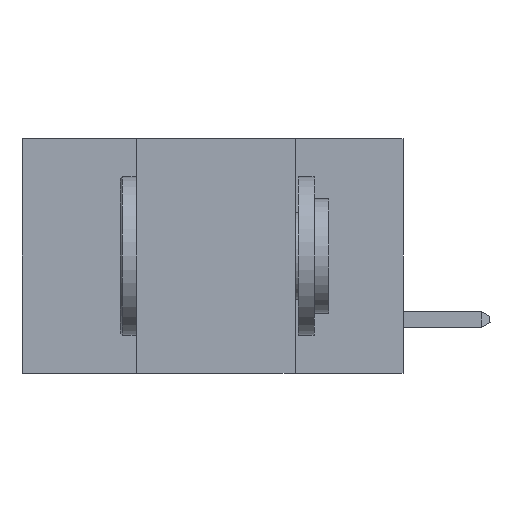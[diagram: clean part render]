
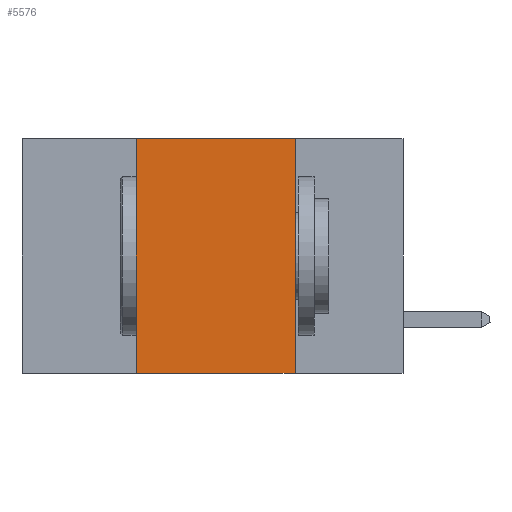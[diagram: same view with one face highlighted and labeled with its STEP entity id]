
A CAD part, left-side view. The second image highlights one B-rep face of the part: STEP entity #5576.
In plain terms, the highlighted planar face has unit normal (-1, 0, 0).
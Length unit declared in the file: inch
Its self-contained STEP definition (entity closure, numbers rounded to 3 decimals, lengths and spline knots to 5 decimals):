
#89 = VERTEX_POINT ( 'NONE', #5878 ) ;
#195 = CARTESIAN_POINT ( 'NONE',  ( 0., 0.6, -0.37 ) ) ;
#388 = VECTOR ( 'NONE', #3309, 39.37008 ) ;
#470 = PLANE ( 'NONE',  #1290 ) ;
#538 = VECTOR ( 'NONE', #8555, 39.37008 ) ;
#962 = LINE ( 'NONE', #195, #388 ) ;
#1290 = AXIS2_PLACEMENT_3D ( 'NONE', #4885, #7760, #3358 ) ;
#1533 = ORIENTED_EDGE ( 'NONE', *, *, #8384, .T. ) ;
#1675 = DIRECTION ( 'NONE',  ( 0., 0., -1. ) ) ;
#1968 = VECTOR ( 'NONE', #2813, 39.37008 ) ;
#2813 = DIRECTION ( 'NONE',  ( 0., -1., 0. ) ) ;
#2861 = VERTEX_POINT ( 'NONE', #6689 ) ;
#2905 = ORIENTED_EDGE ( 'NONE', *, *, #6651, .F. ) ;
#3309 = DIRECTION ( 'NONE',  ( 0., -1., 0. ) ) ;
#3358 = DIRECTION ( 'NONE',  ( 0., 0., -1. ) ) ;
#4235 = EDGE_LOOP ( 'NONE', ( #5993, #7363, #2905, #1533 ) ) ;
#4421 = LINE ( 'NONE', #8132, #1968 ) ;
#4524 = CARTESIAN_POINT ( 'NONE',  ( 0., 0.42, -0.37 ) ) ;
#4829 = CARTESIAN_POINT ( 'NONE',  ( 0., 0.42, 0. ) ) ;
#4885 = CARTESIAN_POINT ( 'NONE',  ( 0., 0.6, 0. ) ) ;
#5033 = VERTEX_POINT ( 'NONE', #4524 ) ;
#5075 = VERTEX_POINT ( 'NONE', #9316 ) ;
#5366 = EDGE_CURVE ( 'NONE', #2861, #89, #7526, .T. ) ;
#5576 = ADVANCED_FACE ( 'NONE', ( #6583 ), #470, .F. ) ;
#5878 = CARTESIAN_POINT ( 'NONE',  ( 0., 0.17, -0.37 ) ) ;
#5993 = ORIENTED_EDGE ( 'NONE', *, *, #5366, .F. ) ;
#6510 = LINE ( 'NONE', #4829, #538 ) ;
#6583 = FACE_OUTER_BOUND ( 'NONE', #4235, .T. ) ;
#6651 = EDGE_CURVE ( 'NONE', #5033, #5075, #6510, .T. ) ;
#6689 = CARTESIAN_POINT ( 'NONE',  ( 0., 0.17, 0. ) ) ;
#7363 = ORIENTED_EDGE ( 'NONE', *, *, #8908, .F. ) ;
#7526 = LINE ( 'NONE', #8982, #9149 ) ;
#7760 = DIRECTION ( 'NONE',  ( 1., 0., 0. ) ) ;
#8132 = CARTESIAN_POINT ( 'NONE',  ( 0., 0.6, 0. ) ) ;
#8384 = EDGE_CURVE ( 'NONE', #5033, #89, #962, .T. ) ;
#8555 = DIRECTION ( 'NONE',  ( 0., 0., 1. ) ) ;
#8908 = EDGE_CURVE ( 'NONE', #5075, #2861, #4421, .T. ) ;
#8982 = CARTESIAN_POINT ( 'NONE',  ( 0., 0.17, 0. ) ) ;
#9149 = VECTOR ( 'NONE', #1675, 39.37008 ) ;
#9316 = CARTESIAN_POINT ( 'NONE',  ( 0., 0.42, 0. ) ) ;
